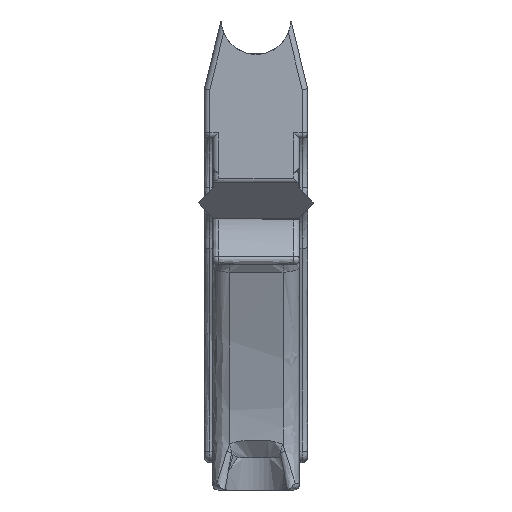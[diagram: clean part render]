
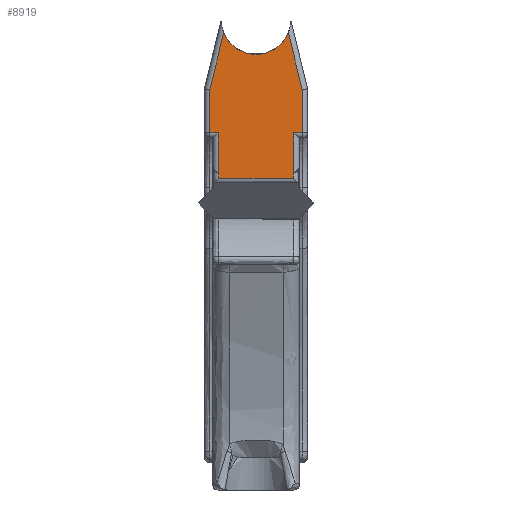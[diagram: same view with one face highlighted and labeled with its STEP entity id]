
A CAD part, front view. The second image highlights one B-rep face of the part: STEP entity #8919.
In plain terms, the highlighted planar face has unit normal (0, -1, 0).
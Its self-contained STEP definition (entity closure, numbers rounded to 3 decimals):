
#941=FACE_OUTER_BOUND('',#1436,.T.);
#1436=EDGE_LOOP('',(#8024,#8025,#8026,#8027,#8028,#8029,#8030,#8031,#8032,
#8033,#8034,#8035,#8036,#8037));
#1648=CIRCLE('',#9521,6.4);
#2452=LINE('',#18873,#3318);
#2463=LINE('',#18900,#3329);
#2473=LINE('',#18917,#3339);
#2485=LINE('',#18946,#3351);
#2486=LINE('',#18949,#3352);
#2487=LINE('',#18951,#3353);
#2488=LINE('',#18953,#3354);
#2489=LINE('',#18955,#3355);
#2490=LINE('',#18959,#3356);
#2491=LINE('',#18961,#3357);
#2492=LINE('',#18962,#3358);
#2493=LINE('',#18964,#3359);
#2494=LINE('',#18965,#3360);
#3318=VECTOR('',#11421,10.);
#3329=VECTOR('',#11448,10.);
#3339=VECTOR('',#11464,10.);
#3351=VECTOR('',#11498,10.);
#3352=VECTOR('',#11501,10.);
#3353=VECTOR('',#11502,10.);
#3354=VECTOR('',#11503,10.);
#3355=VECTOR('',#11504,10.);
#3356=VECTOR('',#11507,10.);
#3357=VECTOR('',#11508,10.);
#3358=VECTOR('',#11509,10.);
#3359=VECTOR('',#11510,1.);
#3360=VECTOR('',#11511,10.);
#4183=VERTEX_POINT('',#18869);
#4185=VERTEX_POINT('',#18872);
#4192=VERTEX_POINT('',#18897);
#4193=VERTEX_POINT('',#18899);
#4197=VERTEX_POINT('',#18916);
#4203=VERTEX_POINT('',#18944);
#4204=VERTEX_POINT('',#18948);
#4205=VERTEX_POINT('',#18950);
#4206=VERTEX_POINT('',#18952);
#4207=VERTEX_POINT('',#18954);
#4208=VERTEX_POINT('',#18956);
#4209=VERTEX_POINT('',#18958);
#4210=VERTEX_POINT('',#18960);
#4211=VERTEX_POINT('',#18963);
#5455=EDGE_CURVE('',#4185,#4183,#2452,.T.);
#5469=EDGE_CURVE('',#4193,#4192,#2463,.T.);
#5480=EDGE_CURVE('',#4193,#4197,#2473,.T.);
#5495=EDGE_CURVE('',#4203,#4192,#2485,.T.);
#5496=EDGE_CURVE('',#4204,#4183,#2486,.T.);
#5497=EDGE_CURVE('',#4205,#4204,#2487,.T.);
#5498=EDGE_CURVE('',#4206,#4205,#2488,.T.);
#5499=EDGE_CURVE('',#4207,#4206,#2489,.T.);
#5500=EDGE_CURVE('',#4207,#4208,#1648,.T.);
#5501=EDGE_CURVE('',#4209,#4208,#2490,.T.);
#5502=EDGE_CURVE('',#4210,#4209,#2491,.T.);
#5503=EDGE_CURVE('',#4197,#4210,#2492,.T.);
#5504=EDGE_CURVE('',#4211,#4203,#2493,.T.);
#5505=EDGE_CURVE('',#4185,#4211,#2494,.T.);
#8024=ORIENTED_EDGE('',*,*,#5496,.F.);
#8025=ORIENTED_EDGE('',*,*,#5497,.F.);
#8026=ORIENTED_EDGE('',*,*,#5498,.F.);
#8027=ORIENTED_EDGE('',*,*,#5499,.F.);
#8028=ORIENTED_EDGE('',*,*,#5500,.T.);
#8029=ORIENTED_EDGE('',*,*,#5501,.F.);
#8030=ORIENTED_EDGE('',*,*,#5502,.F.);
#8031=ORIENTED_EDGE('',*,*,#5503,.F.);
#8032=ORIENTED_EDGE('',*,*,#5480,.F.);
#8033=ORIENTED_EDGE('',*,*,#5469,.T.);
#8034=ORIENTED_EDGE('',*,*,#5495,.F.);
#8035=ORIENTED_EDGE('',*,*,#5504,.F.);
#8036=ORIENTED_EDGE('',*,*,#5505,.F.);
#8037=ORIENTED_EDGE('',*,*,#5455,.T.);
#8462=PLANE('',#9520);
#8919=ADVANCED_FACE('',(#941),#8462,.T.);
#9520=AXIS2_PLACEMENT_3D('',#18947,#11499,#11500);
#9521=AXIS2_PLACEMENT_3D('',#18957,#11505,#11506);
#11421=DIRECTION('',(0.707,0.,0.707));
#11448=DIRECTION('',(0.707,0.,-0.707));
#11464=DIRECTION('',(0.,0.,1.));
#11498=DIRECTION('',(0.,0.,1.));
#11499=DIRECTION('center_axis',(0.,-1.,0.));
#11500=DIRECTION('ref_axis',(1.,0.,0.));
#11501=DIRECTION('',(0.,0.,-1.));
#11502=DIRECTION('',(-1.,0.,0.));
#11503=DIRECTION('',(0.,0.,-1.));
#11504=DIRECTION('',(0.234,0.,-0.972));
#11505=DIRECTION('center_axis',(0.,1.,0.));
#11506=DIRECTION('ref_axis',(1.,0.,0.));
#11507=DIRECTION('',(0.234,0.,0.972));
#11508=DIRECTION('',(0.,0.,1.));
#11509=DIRECTION('',(-1.,0.,0.));
#11510=DIRECTION('',(-1.,0.,0.));
#11511=DIRECTION('',(0.,0.,-1.));
#18869=CARTESIAN_POINT('',(14.9,-169.,-12.));
#18872=CARTESIAN_POINT('',(14.786,-169.,-12.114));
#18873=CARTESIAN_POINT('',(15.3,-169.,-11.6));
#18897=CARTESIAN_POINT('',(1.114,-169.,-12.114));
#18899=CARTESIAN_POINT('',(1.,-169.,-12.));
#18900=CARTESIAN_POINT('',(-3.375,-169.,-7.625));
#18916=CARTESIAN_POINT('',(1.,-169.,-4.6));
#18917=CARTESIAN_POINT('',(1.,-169.,-8.575));
#18944=CARTESIAN_POINT('',(1.114,-169.,-12.908));
#18946=CARTESIAN_POINT('',(1.114,-169.,-6.143));
#18947=CARTESIAN_POINT('Origin',(15.9,-169.,2.25));
#18948=CARTESIAN_POINT('',(14.9,-169.,-4.6));
#18949=CARTESIAN_POINT('',(14.9,-169.,4.475));
#18950=CARTESIAN_POINT('',(16.4,-169.,-4.6));
#18951=CARTESIAN_POINT('',(8.675,-169.,-4.6));
#18952=CARTESIAN_POINT('',(16.4,-169.,3.381));
#18953=CARTESIAN_POINT('',(16.4,-169.,-0.213));
#18954=CARTESIAN_POINT('',(13.888,-169.,13.812));
#18955=CARTESIAN_POINT('',(15.054,-169.,8.971));
#18956=CARTESIAN_POINT('',(2.012,-169.,13.812));
#18957=CARTESIAN_POINT('Origin',(7.95,-169.,16.2));
#18958=CARTESIAN_POINT('',(-0.5,-169.,3.381));
#18959=CARTESIAN_POINT('',(-0.193,-169.,4.655));
#18960=CARTESIAN_POINT('',(-0.5,-169.,-4.6));
#18961=CARTESIAN_POINT('',(-0.5,-169.,-0.213));
#18962=CARTESIAN_POINT('',(8.675,-169.,-4.6));
#18963=CARTESIAN_POINT('',(14.786,-169.,-12.908));
#18964=CARTESIAN_POINT('',(15.786,-169.,-12.908));
#18965=CARTESIAN_POINT('',(14.786,-169.,-4.375));
